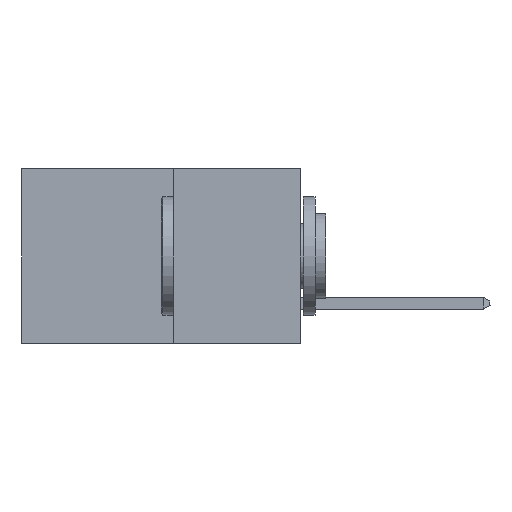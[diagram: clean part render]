
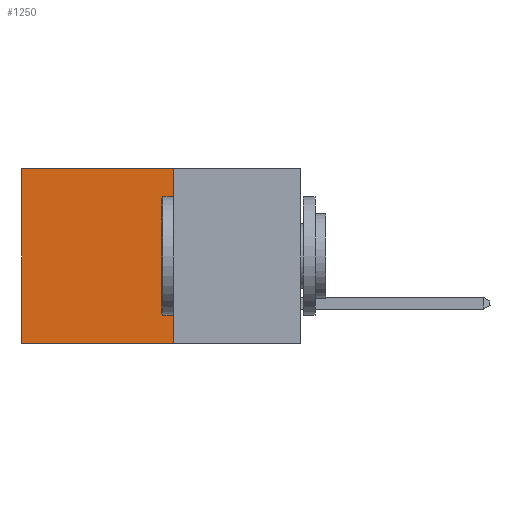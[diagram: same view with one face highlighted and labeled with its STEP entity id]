
A CAD part, left-side view. The second image highlights one B-rep face of the part: STEP entity #1250.
In plain terms, the highlighted planar face has unit normal (-1, 0, 0).
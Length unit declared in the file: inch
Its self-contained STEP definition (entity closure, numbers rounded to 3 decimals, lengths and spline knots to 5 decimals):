
#509 = PLANE ( 'NONE',  #19779 ) ;
#1250 = ADVANCED_FACE ( 'NONE', ( #2793 ), #509, .F. ) ;
#2793 = FACE_OUTER_BOUND ( 'NONE', #9599, .T. ) ;
#4011 = CARTESIAN_POINT ( 'NONE',  ( 0.277, 0.27, -0.37 ) ) ;
#4085 = EDGE_CURVE ( 'NONE', #20378, #30684, #12830, .T. ) ;
#5033 = ORIENTED_EDGE ( 'NONE', *, *, #4085, .F. ) ;
#5363 = DIRECTION ( 'NONE',  ( 0., 0., -1. ) ) ;
#5708 = VERTEX_POINT ( 'NONE', #12306 ) ;
#5756 = DIRECTION ( 'NONE',  ( 0., 1., 0. ) ) ;
#6576 = CARTESIAN_POINT ( 'NONE',  ( 0.277, 0.27, -0.37 ) ) ;
#7257 = CARTESIAN_POINT ( 'NONE',  ( 0.277, 0.59, -0.37 ) ) ;
#7692 = VECTOR ( 'NONE', #5756, 39.37008 ) ;
#7835 = EDGE_CURVE ( 'NONE', #5708, #22854, #26116, .T. ) ;
#8835 = CARTESIAN_POINT ( 'NONE',  ( 0.277, 0.59, -0.37 ) ) ;
#9599 = EDGE_LOOP ( 'NONE', ( #26294, #5033, #12042, #26482 ) ) ;
#10430 = LINE ( 'NONE', #15380, #27811 ) ;
#11776 = EDGE_CURVE ( 'NONE', #5708, #20378, #10430, .T. ) ;
#12042 = ORIENTED_EDGE ( 'NONE', *, *, #11776, .F. ) ;
#12306 = CARTESIAN_POINT ( 'NONE',  ( 0.277, 0.27, 0. ) ) ;
#12830 = LINE ( 'NONE', #6576, #7692 ) ;
#12997 = VECTOR ( 'NONE', #21047, 39.37008 ) ;
#14293 = EDGE_CURVE ( 'NONE', #22854, #30684, #23444, .T. ) ;
#15380 = CARTESIAN_POINT ( 'NONE',  ( 0.277, 0.27, -0.37 ) ) ;
#15692 = DIRECTION ( 'NONE',  ( 0., 0., -1. ) ) ;
#15847 = CARTESIAN_POINT ( 'NONE',  ( 0.277, 0.59, 0. ) ) ;
#17785 = CARTESIAN_POINT ( 'NONE',  ( 0.277, 0.27, -0.37 ) ) ;
#17818 = DIRECTION ( 'NONE',  ( 1., 0., 0. ) ) ;
#19779 = AXIS2_PLACEMENT_3D ( 'NONE', #17785, #17818, #15692 ) ;
#20378 = VERTEX_POINT ( 'NONE', #4011 ) ;
#21047 = DIRECTION ( 'NONE',  ( 0., 1., 0. ) ) ;
#21293 = DIRECTION ( 'NONE',  ( 0., 0., -1. ) ) ;
#22687 = VECTOR ( 'NONE', #21293, 39.37008 ) ;
#22854 = VERTEX_POINT ( 'NONE', #15847 ) ;
#23444 = LINE ( 'NONE', #8835, #22687 ) ;
#23479 = CARTESIAN_POINT ( 'NONE',  ( 0.277, 0.27, 0. ) ) ;
#26116 = LINE ( 'NONE', #23479, #12997 ) ;
#26294 = ORIENTED_EDGE ( 'NONE', *, *, #14293, .T. ) ;
#26482 = ORIENTED_EDGE ( 'NONE', *, *, #7835, .T. ) ;
#27811 = VECTOR ( 'NONE', #5363, 39.37008 ) ;
#30684 = VERTEX_POINT ( 'NONE', #7257 ) ;
